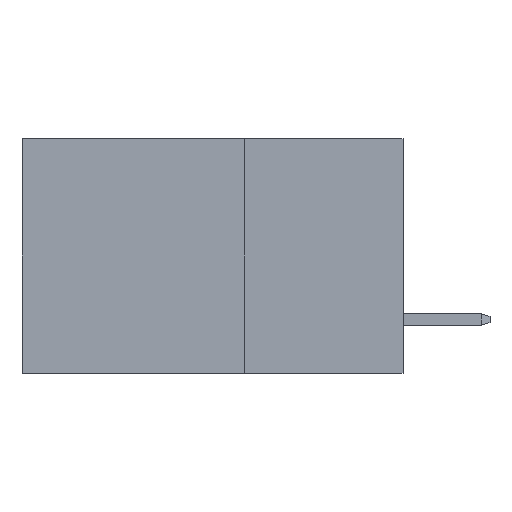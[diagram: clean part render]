
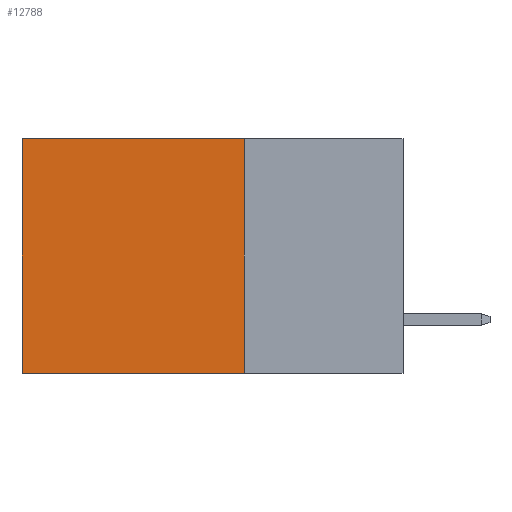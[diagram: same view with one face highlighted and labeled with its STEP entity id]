
A CAD part, left-side view. The second image highlights one B-rep face of the part: STEP entity #12788.
In plain terms, the highlighted planar face has unit normal (-1, 0, 0).
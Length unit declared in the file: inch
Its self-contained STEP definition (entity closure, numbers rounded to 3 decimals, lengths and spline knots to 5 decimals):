
#414 = CARTESIAN_POINT ( 'NONE',  ( 0.2875, 0.6, -0.37 ) ) ;
#606 = VERTEX_POINT ( 'NONE', #6176 ) ;
#957 = LINE ( 'NONE', #10480, #12077 ) ;
#1521 = DIRECTION ( 'NONE',  ( 1., 0., 0. ) ) ;
#2077 = VECTOR ( 'NONE', #2534, 39.37008 ) ;
#2308 = VERTEX_POINT ( 'NONE', #2948 ) ;
#2424 = EDGE_LOOP ( 'NONE', ( #12758, #13078, #2573, #5257 ) ) ;
#2437 = LINE ( 'NONE', #5859, #3129 ) ;
#2534 = DIRECTION ( 'NONE',  ( 0., 0., -1. ) ) ;
#2573 = ORIENTED_EDGE ( 'NONE', *, *, #4350, .F. ) ;
#2948 = CARTESIAN_POINT ( 'NONE',  ( 0.2875, 0.25, 0. ) ) ;
#3129 = VECTOR ( 'NONE', #10096, 39.37008 ) ;
#3408 = VERTEX_POINT ( 'NONE', #7633 ) ;
#3755 = PLANE ( 'NONE',  #6753 ) ;
#4350 = EDGE_CURVE ( 'NONE', #2308, #606, #2437, .T. ) ;
#4556 = LINE ( 'NONE', #6588, #2077 ) ;
#5158 = CARTESIAN_POINT ( 'NONE',  ( 0.2875, 0.25, 0. ) ) ;
#5257 = ORIENTED_EDGE ( 'NONE', *, *, #10738, .T. ) ;
#5481 = DIRECTION ( 'NONE',  ( 0., 1., 0. ) ) ;
#5774 = DIRECTION ( 'NONE',  ( 0., 0., -1. ) ) ;
#5820 = VECTOR ( 'NONE', #12540, 39.37008 ) ;
#5859 = CARTESIAN_POINT ( 'NONE',  ( 0.2875, 0.25, 0. ) ) ;
#6176 = CARTESIAN_POINT ( 'NONE',  ( 0.2875, 0.25, -0.37 ) ) ;
#6360 = EDGE_CURVE ( 'NONE', #606, #11073, #957, .T. ) ;
#6588 = CARTESIAN_POINT ( 'NONE',  ( 0.2875, 0.6, 0. ) ) ;
#6753 = AXIS2_PLACEMENT_3D ( 'NONE', #11203, #1521, #5774 ) ;
#6903 = EDGE_CURVE ( 'NONE', #3408, #11073, #4556, .T. ) ;
#7633 = CARTESIAN_POINT ( 'NONE',  ( 0.2875, 0.6, 0. ) ) ;
#10096 = DIRECTION ( 'NONE',  ( 0., 0., -1. ) ) ;
#10159 = FACE_OUTER_BOUND ( 'NONE', #2424, .T. ) ;
#10480 = CARTESIAN_POINT ( 'NONE',  ( 0.2875, 0.25, -0.37 ) ) ;
#10738 = EDGE_CURVE ( 'NONE', #2308, #3408, #13582, .T. ) ;
#11073 = VERTEX_POINT ( 'NONE', #414 ) ;
#11203 = CARTESIAN_POINT ( 'NONE',  ( 0.2875, 0.25, 0. ) ) ;
#12077 = VECTOR ( 'NONE', #5481, 39.37008 ) ;
#12540 = DIRECTION ( 'NONE',  ( 0., 1., 0. ) ) ;
#12758 = ORIENTED_EDGE ( 'NONE', *, *, #6903, .T. ) ;
#12788 = ADVANCED_FACE ( 'NONE', ( #10159 ), #3755, .F. ) ;
#13078 = ORIENTED_EDGE ( 'NONE', *, *, #6360, .F. ) ;
#13582 = LINE ( 'NONE', #5158, #5820 ) ;
